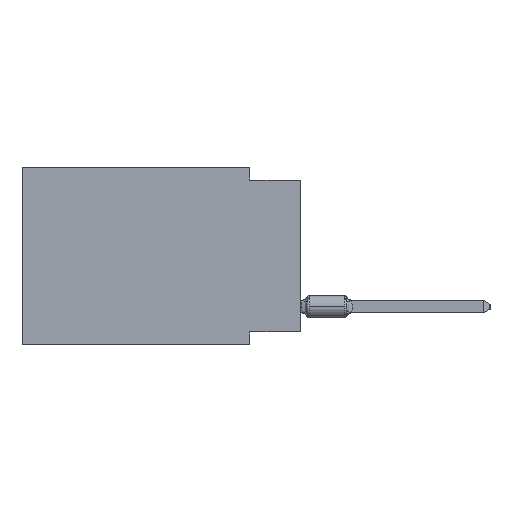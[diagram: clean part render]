
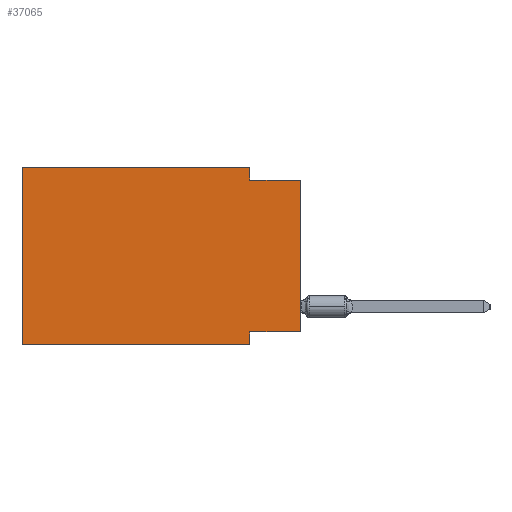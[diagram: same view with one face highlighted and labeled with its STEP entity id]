
A CAD part, left-side view. The second image highlights one B-rep face of the part: STEP entity #37065.
In plain terms, the highlighted planar face has unit normal (-1, 0, 0).
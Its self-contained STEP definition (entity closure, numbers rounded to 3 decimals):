
#341 = VERTEX_POINT ( 'NONE', #3187 ) ;
#689 = DIRECTION ( 'NONE',  ( 0., 0., 1. ) ) ;
#863 = CARTESIAN_POINT ( 'NONE',  ( 0., 2.54, -8.89 ) ) ;
#1056 = CARTESIAN_POINT ( 'NONE',  ( 0., 0., -0.635 ) ) ;
#1110 = VERTEX_POINT ( 'NONE', #36963 ) ;
#1233 = DIRECTION ( 'NONE',  ( 0., 0., -1. ) ) ;
#2510 = ORIENTED_EDGE ( 'NONE', *, *, #40673, .T. ) ;
#2978 = DIRECTION ( 'NONE',  ( 0., 0., 1. ) ) ;
#3187 = CARTESIAN_POINT ( 'NONE',  ( 0., 0., -8.255 ) ) ;
#3798 = CARTESIAN_POINT ( 'NONE',  ( 0., 0., -0.635 ) ) ;
#5170 = ORIENTED_EDGE ( 'NONE', *, *, #22314, .F. ) ;
#5528 = EDGE_CURVE ( 'NONE', #1110, #28814, #27663, .T. ) ;
#9630 = VERTEX_POINT ( 'NONE', #36841 ) ;
#10210 = LINE ( 'NONE', #16281, #36804 ) ;
#10708 = ORIENTED_EDGE ( 'NONE', *, *, #22979, .T. ) ;
#11218 = CARTESIAN_POINT ( 'NONE',  ( 0., 2.54, -8.255 ) ) ;
#12362 = CARTESIAN_POINT ( 'NONE',  ( 0., 2.54, -8.89 ) ) ;
#12507 = ORIENTED_EDGE ( 'NONE', *, *, #5528, .F. ) ;
#12678 = AXIS2_PLACEMENT_3D ( 'NONE', #38041, #31099, #1233 ) ;
#13073 = EDGE_LOOP ( 'NONE', ( #10708, #5170, #12507, #19869, #36557, #2510, #35537, #37420 ) ) ;
#13098 = CARTESIAN_POINT ( 'NONE',  ( 0., 2.54, -0.635 ) ) ;
#13820 = DIRECTION ( 'NONE',  ( 0., 0., -1. ) ) ;
#14241 = CARTESIAN_POINT ( 'NONE',  ( 0., 2.54, 0. ) ) ;
#15630 = DIRECTION ( 'NONE',  ( 0., -1., 0. ) ) ;
#15980 = CARTESIAN_POINT ( 'NONE',  ( 0., 13.97, 0. ) ) ;
#16281 = CARTESIAN_POINT ( 'NONE',  ( 0., 0., -8.255 ) ) ;
#16327 = VECTOR ( 'NONE', #15630, 1000. ) ;
#16835 = VECTOR ( 'NONE', #40530, 1000. ) ;
#17298 = LINE ( 'NONE', #1056, #24363 ) ;
#19869 = ORIENTED_EDGE ( 'NONE', *, *, #29269, .F. ) ;
#20136 = LINE ( 'NONE', #863, #22160 ) ;
#21673 = VERTEX_POINT ( 'NONE', #25736 ) ;
#21801 = FACE_OUTER_BOUND ( 'NONE', #13073, .T. ) ;
#22160 = VECTOR ( 'NONE', #29672, 1000. ) ;
#22314 = EDGE_CURVE ( 'NONE', #28814, #34450, #17298, .T. ) ;
#22752 = LINE ( 'NONE', #29492, #16327 ) ;
#22979 = EDGE_CURVE ( 'NONE', #341, #34450, #26896, .T. ) ;
#23070 = VECTOR ( 'NONE', #2978, 1000. ) ;
#24363 = VECTOR ( 'NONE', #27057, 1000. ) ;
#25736 = CARTESIAN_POINT ( 'NONE',  ( 0., 13.97, -8.89 ) ) ;
#26896 = LINE ( 'NONE', #33179, #33434 ) ;
#27057 = DIRECTION ( 'NONE',  ( 0., -1., 0. ) ) ;
#27334 = CARTESIAN_POINT ( 'NONE',  ( 0., 13.97, 0. ) ) ;
#27663 = LINE ( 'NONE', #14241, #42780 ) ;
#28306 = EDGE_CURVE ( 'NONE', #21673, #9630, #32658, .T. ) ;
#28814 = VERTEX_POINT ( 'NONE', #13098 ) ;
#29269 = EDGE_CURVE ( 'NONE', #9630, #1110, #33611, .T. ) ;
#29492 = CARTESIAN_POINT ( 'NONE',  ( 0., 13.97, -8.89 ) ) ;
#29672 = DIRECTION ( 'NONE',  ( 0., 0., -1. ) ) ;
#31099 = DIRECTION ( 'NONE',  ( 1., 0., 0. ) ) ;
#31753 = VERTEX_POINT ( 'NONE', #11218 ) ;
#32658 = LINE ( 'NONE', #15980, #23070 ) ;
#33179 = CARTESIAN_POINT ( 'NONE',  ( 0., 0., 0. ) ) ;
#33434 = VECTOR ( 'NONE', #689, 1000. ) ;
#33611 = LINE ( 'NONE', #27334, #16835 ) ;
#34028 = EDGE_CURVE ( 'NONE', #31753, #35143, #20136, .T. ) ;
#34450 = VERTEX_POINT ( 'NONE', #3798 ) ;
#35143 = VERTEX_POINT ( 'NONE', #12362 ) ;
#35537 = ORIENTED_EDGE ( 'NONE', *, *, #34028, .F. ) ;
#36557 = ORIENTED_EDGE ( 'NONE', *, *, #28306, .F. ) ;
#36634 = DIRECTION ( 'NONE',  ( 0., 1., 0. ) ) ;
#36804 = VECTOR ( 'NONE', #36634, 1000. ) ;
#36841 = CARTESIAN_POINT ( 'NONE',  ( 0., 13.97, 0. ) ) ;
#36963 = CARTESIAN_POINT ( 'NONE',  ( 0., 2.54, 0. ) ) ;
#37065 = ADVANCED_FACE ( 'NONE', ( #21801 ), #37822, .F. ) ;
#37420 = ORIENTED_EDGE ( 'NONE', *, *, #42317, .F. ) ;
#37822 = PLANE ( 'NONE',  #12678 ) ;
#38041 = CARTESIAN_POINT ( 'NONE',  ( 0., 13.97, 0. ) ) ;
#40530 = DIRECTION ( 'NONE',  ( 0., -1., 0. ) ) ;
#40673 = EDGE_CURVE ( 'NONE', #21673, #35143, #22752, .T. ) ;
#42317 = EDGE_CURVE ( 'NONE', #341, #31753, #10210, .T. ) ;
#42780 = VECTOR ( 'NONE', #13820, 1000. ) ;
